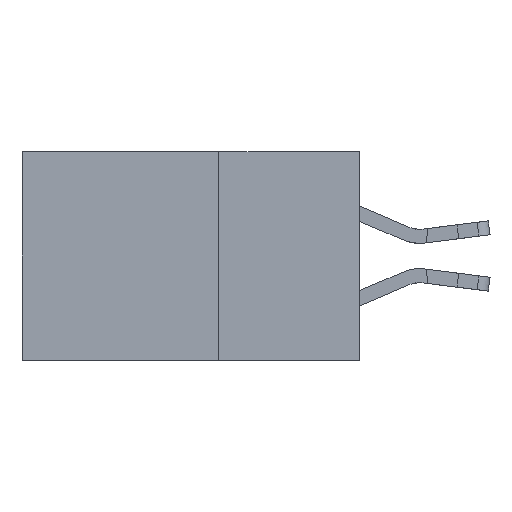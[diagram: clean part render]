
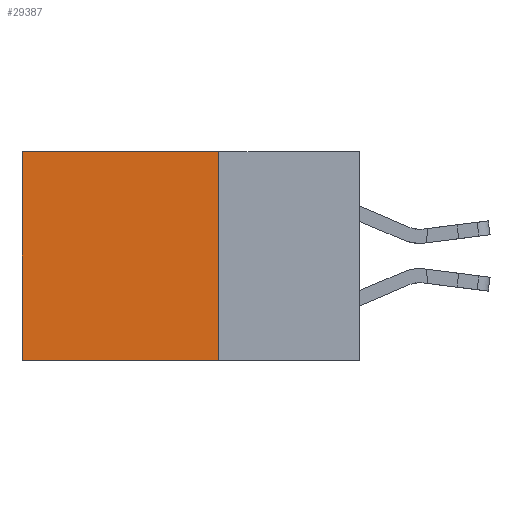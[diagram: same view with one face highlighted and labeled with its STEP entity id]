
A CAD part, left-side view. The second image highlights one B-rep face of the part: STEP entity #29387.
In plain terms, the highlighted planar face has unit normal (-1, 0, 0).
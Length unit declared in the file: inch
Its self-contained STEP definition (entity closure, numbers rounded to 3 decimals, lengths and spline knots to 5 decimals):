
#802 = CARTESIAN_POINT ( 'NONE',  ( 0.2875, 0.6, 0. ) ) ;
#1526 = LINE ( 'NONE', #24784, #33689 ) ;
#2560 = AXIS2_PLACEMENT_3D ( 'NONE', #28603, #26243, #10290 ) ;
#2725 = FACE_OUTER_BOUND ( 'NONE', #8701, .T. ) ;
#3941 = EDGE_CURVE ( 'NONE', #5111, #24801, #1526, .T. ) ;
#4552 = CARTESIAN_POINT ( 'NONE',  ( 0.2875, 0.25, 0. ) ) ;
#5111 = VERTEX_POINT ( 'NONE', #802 ) ;
#5548 = VERTEX_POINT ( 'NONE', #31008 ) ;
#7622 = PLANE ( 'NONE',  #2560 ) ;
#8501 = LINE ( 'NONE', #11926, #28947 ) ;
#8593 = ORIENTED_EDGE ( 'NONE', *, *, #26974, .F. ) ;
#8701 = EDGE_LOOP ( 'NONE', ( #19630, #22892, #8593, #18137 ) ) ;
#10290 = DIRECTION ( 'NONE',  ( 0., 0., -1. ) ) ;
#11926 = CARTESIAN_POINT ( 'NONE',  ( 0.2875, 0.25, -0.37 ) ) ;
#12155 = DIRECTION ( 'NONE',  ( 0., 1., 0. ) ) ;
#15080 = CARTESIAN_POINT ( 'NONE',  ( 0.2875, 0.6, -0.37 ) ) ;
#15330 = VERTEX_POINT ( 'NONE', #15793 ) ;
#15793 = CARTESIAN_POINT ( 'NONE',  ( 0.2875, 0.25, -0.37 ) ) ;
#15860 = EDGE_CURVE ( 'NONE', #5548, #5111, #21796, .T. ) ;
#15928 = DIRECTION ( 'NONE',  ( 0., 0., -1. ) ) ;
#16020 = VECTOR ( 'NONE', #31534, 39.37008 ) ;
#16368 = CARTESIAN_POINT ( 'NONE',  ( 0.2875, 0.25, 0. ) ) ;
#18137 = ORIENTED_EDGE ( 'NONE', *, *, #15860, .T. ) ;
#19630 = ORIENTED_EDGE ( 'NONE', *, *, #3941, .T. ) ;
#21796 = LINE ( 'NONE', #4552, #16020 ) ;
#22892 = ORIENTED_EDGE ( 'NONE', *, *, #30293, .F. ) ;
#24261 = DIRECTION ( 'NONE',  ( 0., 0., -1. ) ) ;
#24533 = LINE ( 'NONE', #16368, #32946 ) ;
#24784 = CARTESIAN_POINT ( 'NONE',  ( 0.2875, 0.6, 0. ) ) ;
#24801 = VERTEX_POINT ( 'NONE', #15080 ) ;
#26243 = DIRECTION ( 'NONE',  ( 1., 0., 0. ) ) ;
#26974 = EDGE_CURVE ( 'NONE', #5548, #15330, #24533, .T. ) ;
#28603 = CARTESIAN_POINT ( 'NONE',  ( 0.2875, 0.25, 0. ) ) ;
#28947 = VECTOR ( 'NONE', #12155, 39.37008 ) ;
#29387 = ADVANCED_FACE ( 'NONE', ( #2725 ), #7622, .F. ) ;
#30293 = EDGE_CURVE ( 'NONE', #15330, #24801, #8501, .T. ) ;
#31008 = CARTESIAN_POINT ( 'NONE',  ( 0.2875, 0.25, 0. ) ) ;
#31534 = DIRECTION ( 'NONE',  ( 0., 1., 0. ) ) ;
#32946 = VECTOR ( 'NONE', #24261, 39.37008 ) ;
#33689 = VECTOR ( 'NONE', #15928, 39.37008 ) ;
